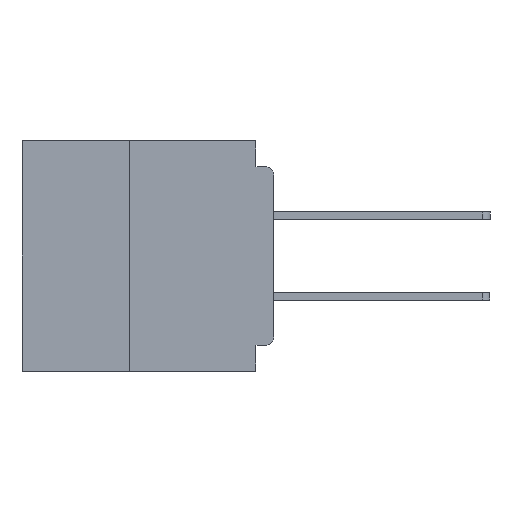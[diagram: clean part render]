
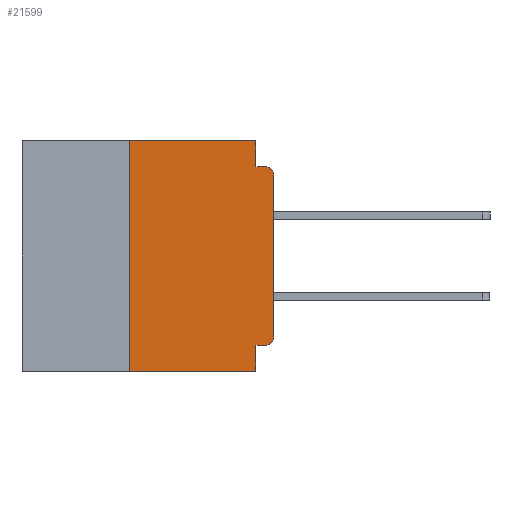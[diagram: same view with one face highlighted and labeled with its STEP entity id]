
A CAD part, left-side view. The second image highlights one B-rep face of the part: STEP entity #21599.
In plain terms, the highlighted planar face has unit normal (-1, 0, 0).
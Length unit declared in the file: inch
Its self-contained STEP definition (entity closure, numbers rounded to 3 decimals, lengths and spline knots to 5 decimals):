
#613 = VERTEX_POINT ( 'NONE', #1007 ) ;
#700 = CARTESIAN_POINT ( 'NONE',  ( 0., 0.25, 0. ) ) ;
#1007 = CARTESIAN_POINT ( 'NONE',  ( 0., 0.25, -0.4 ) ) ;
#1133 = EDGE_CURVE ( 'NONE', #7800, #23501, #14570, .T. ) ;
#1634 = ORIENTED_EDGE ( 'NONE', *, *, #20225, .F. ) ;
#2291 = EDGE_CURVE ( 'NONE', #23501, #30068, #24377, .T. ) ;
#4675 = VECTOR ( 'NONE', #20817, 39.37008 ) ;
#5161 = AXIS2_PLACEMENT_3D ( 'NONE', #7477, #36762, #17379 ) ;
#5463 = CARTESIAN_POINT ( 'NONE',  ( 0., 0.031, 0. ) ) ;
#5667 = DIRECTION ( 'NONE',  ( 0., -1., 0. ) ) ;
#6108 = ORIENTED_EDGE ( 'NONE', *, *, #6754, .T. ) ;
#6177 = EDGE_CURVE ( 'NONE', #18717, #6953, #28669, .T. ) ;
#6432 = DIRECTION ( 'NONE',  ( 0., -1., 0. ) ) ;
#6604 = ORIENTED_EDGE ( 'NONE', *, *, #31328, .F. ) ;
#6754 = EDGE_CURVE ( 'NONE', #9158, #22849, #15965, .T. ) ;
#6953 = VERTEX_POINT ( 'NONE', #9061 ) ;
#7245 = DIRECTION ( 'NONE',  ( 0., 1., 0. ) ) ;
#7477 = CARTESIAN_POINT ( 'NONE',  ( 0., 0.437, 0. ) ) ;
#7728 = CARTESIAN_POINT ( 'NONE',  ( 0., 0., -0.06 ) ) ;
#7800 = VERTEX_POINT ( 'NONE', #700 ) ;
#8203 = DIRECTION ( 'NONE',  ( -1., 0., 0. ) ) ;
#8617 = ORIENTED_EDGE ( 'NONE', *, *, #2291, .F. ) ;
#8939 = VECTOR ( 'NONE', #6432, 39.37008 ) ;
#9007 = ORIENTED_EDGE ( 'NONE', *, *, #1133, .F. ) ;
#9061 = CARTESIAN_POINT ( 'NONE',  ( 0., 0., -0.34 ) ) ;
#9158 = VERTEX_POINT ( 'NONE', #7728 ) ;
#9654 = EDGE_CURVE ( 'NONE', #40740, #33079, #40164, .T. ) ;
#9717 = CARTESIAN_POINT ( 'NONE',  ( 0., 0.015, -0.34 ) ) ;
#9981 = VECTOR ( 'NONE', #5667, 39.37008 ) ;
#10777 = PLANE ( 'NONE',  #5161 ) ;
#10936 = LINE ( 'NONE', #18175, #26216 ) ;
#10958 = VECTOR ( 'NONE', #7245, 39.37008 ) ;
#10967 = EDGE_CURVE ( 'NONE', #6953, #9158, #38031, .T. ) ;
#11271 = FACE_OUTER_BOUND ( 'NONE', #26356, .T. ) ;
#12807 = EDGE_CURVE ( 'NONE', #613, #7800, #10936, .T. ) ;
#13044 = DIRECTION ( 'NONE',  ( 0., 0., -1. ) ) ;
#13310 = VECTOR ( 'NONE', #22047, 39.37008 ) ;
#14570 = LINE ( 'NONE', #25986, #8939 ) ;
#15965 = CIRCLE ( 'NONE', #25714, 0.015 ) ;
#17379 = DIRECTION ( 'NONE',  ( 0., 0., -1. ) ) ;
#17421 = CARTESIAN_POINT ( 'NONE',  ( 0., 0.015, -0.045 ) ) ;
#18175 = CARTESIAN_POINT ( 'NONE',  ( 0., 0.25, -0.4 ) ) ;
#18717 = VERTEX_POINT ( 'NONE', #22653 ) ;
#19704 = LINE ( 'NONE', #28500, #9981 ) ;
#20225 = EDGE_CURVE ( 'NONE', #30068, #22849, #21090, .T. ) ;
#20657 = LINE ( 'NONE', #30030, #10958 ) ;
#20817 = DIRECTION ( 'NONE',  ( 0., -1., 0. ) ) ;
#21090 = LINE ( 'NONE', #40205, #4675 ) ;
#21599 = ADVANCED_FACE ( 'NONE', ( #11271 ), #10777, .F. ) ;
#21934 = DIRECTION ( 'NONE',  ( 0., 0., -1. ) ) ;
#21980 = ORIENTED_EDGE ( 'NONE', *, *, #6177, .T. ) ;
#22047 = DIRECTION ( 'NONE',  ( 0., 0., -1. ) ) ;
#22653 = CARTESIAN_POINT ( 'NONE',  ( 0., 0.015, -0.355 ) ) ;
#22849 = VERTEX_POINT ( 'NONE', #17421 ) ;
#23501 = VERTEX_POINT ( 'NONE', #40284 ) ;
#23999 = CARTESIAN_POINT ( 'NONE',  ( 0., 0.031, -0.4 ) ) ;
#24377 = LINE ( 'NONE', #5463, #35015 ) ;
#24555 = ORIENTED_EDGE ( 'NONE', *, *, #37150, .T. ) ;
#25714 = AXIS2_PLACEMENT_3D ( 'NONE', #27693, #8203, #30946 ) ;
#25986 = CARTESIAN_POINT ( 'NONE',  ( 0., 0.437, 0. ) ) ;
#26216 = VECTOR ( 'NONE', #27622, 39.37008 ) ;
#26356 = EDGE_LOOP ( 'NONE', ( #28240, #6108, #1634, #8617, #9007, #29310, #24555, #28741, #6604, #21980 ) ) ;
#27622 = DIRECTION ( 'NONE',  ( 0., 0., 1. ) ) ;
#27693 = CARTESIAN_POINT ( 'NONE',  ( 0., 0.015, -0.06 ) ) ;
#28240 = ORIENTED_EDGE ( 'NONE', *, *, #10967, .T. ) ;
#28500 = CARTESIAN_POINT ( 'NONE',  ( 0., 0.437, -0.4 ) ) ;
#28669 = CIRCLE ( 'NONE', #36009, 0.015 ) ;
#28741 = ORIENTED_EDGE ( 'NONE', *, *, #9654, .F. ) ;
#29310 = ORIENTED_EDGE ( 'NONE', *, *, #12807, .F. ) ;
#29424 = VECTOR ( 'NONE', #31717, 39.37008 ) ;
#30030 = CARTESIAN_POINT ( 'NONE',  ( 0., 0., -0.355 ) ) ;
#30068 = VERTEX_POINT ( 'NONE', #36768 ) ;
#30946 = DIRECTION ( 'NONE',  ( 0., 0., -1. ) ) ;
#31328 = EDGE_CURVE ( 'NONE', #18717, #40740, #20657, .T. ) ;
#31717 = DIRECTION ( 'NONE',  ( 0., 0., 1. ) ) ;
#32491 = DIRECTION ( 'NONE',  ( -1., 0., 0. ) ) ;
#33079 = VERTEX_POINT ( 'NONE', #23999 ) ;
#34690 = CARTESIAN_POINT ( 'NONE',  ( 0., 0., 0. ) ) ;
#35015 = VECTOR ( 'NONE', #21934, 39.37008 ) ;
#36009 = AXIS2_PLACEMENT_3D ( 'NONE', #9717, #32491, #13044 ) ;
#36762 = DIRECTION ( 'NONE',  ( 1., 0., 0. ) ) ;
#36768 = CARTESIAN_POINT ( 'NONE',  ( 0., 0.031, -0.045 ) ) ;
#37150 = EDGE_CURVE ( 'NONE', #613, #33079, #19704, .T. ) ;
#38031 = LINE ( 'NONE', #34690, #29424 ) ;
#38181 = CARTESIAN_POINT ( 'NONE',  ( 0., 0.031, -0.4 ) ) ;
#40164 = LINE ( 'NONE', #38181, #13310 ) ;
#40205 = CARTESIAN_POINT ( 'NONE',  ( 0., 0., -0.045 ) ) ;
#40284 = CARTESIAN_POINT ( 'NONE',  ( 0., 0.031, 0. ) ) ;
#40474 = CARTESIAN_POINT ( 'NONE',  ( 0., 0.031, -0.355 ) ) ;
#40740 = VERTEX_POINT ( 'NONE', #40474 ) ;
